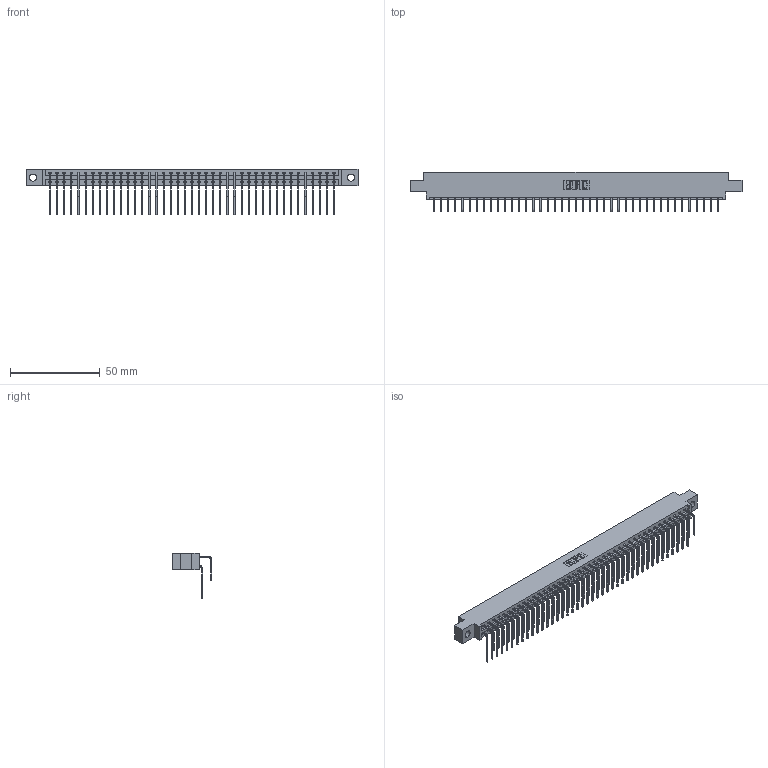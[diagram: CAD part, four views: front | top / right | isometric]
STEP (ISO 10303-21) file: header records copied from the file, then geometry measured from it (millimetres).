
FILE_DESCRIPTION (( 'STEP AP203' ), '1' );
FILE_NAME ('337-082-558-804.STEP', '2019-10-15T17:32:30', ( '' ), ( '' ), 'SwSTEP 2.0', 'SolidWorks 2016', '' );
FILE_SCHEMA (( 'CONFIG_CONTROL_DESIGN' ));
Length unit declared in the file: inch
Products named in the file (4): 337 Part_0.170 Offset - 0.156 Dia-TH; 345-292-001_558 Tail - 2; 345-292-001_558 559 Tail - 1; 337-082-558-804
Assembly tree (83 placements, depth 2):
  337-082-558-804
    337 Part_0.170 Offset - 0.156 Dia-TH
    345-292-001_558 559 Tail - 1  x41
    345-292-001_558 Tail - 2  x41
Bounding box: 185.47 x 22.17 x 25.53 mm (x, y, z)
Volume: 19800.7 mm3; surface area: 24655.5 mm2
Topology: 83 solids, 83 shells, 4710 faces, 14017 edges, 9234 vertices
Faces by surface type: plane 3354, cylinder 1356
Entity records: 33837 total; most frequent: CARTESIAN_POINT 5749, ORIENTED_EDGE 5634, DIRECTION 4873, EDGE_CURVE 2817, VECTOR 2649, LINE 2649, VERTEX_POINT 1874, AXIS2_PLACEMENT_3D 1112
